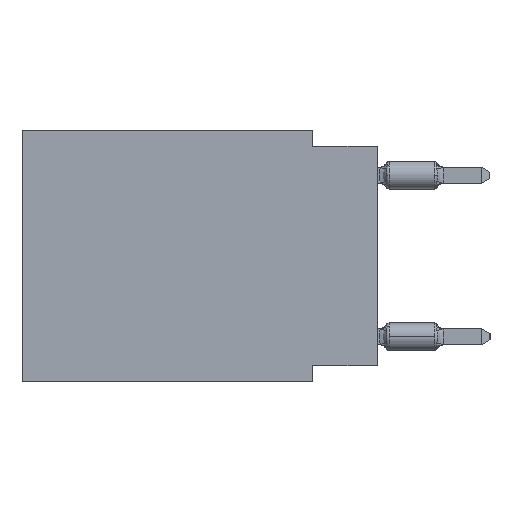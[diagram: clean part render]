
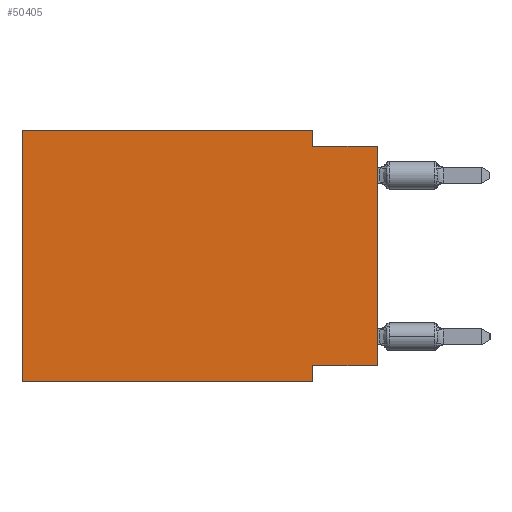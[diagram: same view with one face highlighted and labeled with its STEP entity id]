
A CAD part, left-side view. The second image highlights one B-rep face of the part: STEP entity #50405.
In plain terms, the highlighted planar face has unit normal (-1, 0, 0).
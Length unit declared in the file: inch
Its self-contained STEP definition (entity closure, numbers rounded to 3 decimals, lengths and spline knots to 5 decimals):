
#740 = LINE ( 'NONE', #37298, #24506 ) ;
#2675 = VERTEX_POINT ( 'NONE', #20444 ) ;
#2811 = LINE ( 'NONE', #47509, #9382 ) ;
#3661 = VECTOR ( 'NONE', #38894, 39.37008 ) ;
#3793 = AXIS2_PLACEMENT_3D ( 'NONE', #50603, #45215, #8955 ) ;
#4601 = CARTESIAN_POINT ( 'NONE',  ( 0., 0.1, -0.365 ) ) ;
#4885 = ORIENTED_EDGE ( 'NONE', *, *, #9253, .F. ) ;
#5170 = VERTEX_POINT ( 'NONE', #11547 ) ;
#7883 = CARTESIAN_POINT ( 'NONE',  ( 0., 0.55, -0.39 ) ) ;
#8901 = CARTESIAN_POINT ( 'NONE',  ( 0., 0.1, -0.39 ) ) ;
#8955 = DIRECTION ( 'NONE',  ( 0., 0., -1. ) ) ;
#9253 = EDGE_CURVE ( 'NONE', #12765, #47772, #740, .T. ) ;
#9382 = VECTOR ( 'NONE', #33998, 39.37008 ) ;
#9494 = CARTESIAN_POINT ( 'NONE',  ( 0., 0.1, -0.025 ) ) ;
#11457 = EDGE_CURVE ( 'NONE', #49634, #58229, #49666, .T. ) ;
#11547 = CARTESIAN_POINT ( 'NONE',  ( 0., 0.1, 0. ) ) ;
#11613 = LINE ( 'NONE', #34095, #3661 ) ;
#12765 = VERTEX_POINT ( 'NONE', #9494 ) ;
#13258 = ORIENTED_EDGE ( 'NONE', *, *, #39959, .F. ) ;
#14235 = DIRECTION ( 'NONE',  ( 0., -1., 0. ) ) ;
#15120 = ORIENTED_EDGE ( 'NONE', *, *, #53419, .F. ) ;
#18534 = EDGE_CURVE ( 'NONE', #46167, #5170, #40660, .T. ) ;
#20444 = CARTESIAN_POINT ( 'NONE',  ( 0., 0.55, -0.39 ) ) ;
#20873 = CARTESIAN_POINT ( 'NONE',  ( 0., 0.55, 0. ) ) ;
#21294 = ORIENTED_EDGE ( 'NONE', *, *, #44246, .T. ) ;
#23022 = PLANE ( 'NONE',  #3793 ) ;
#23201 = ORIENTED_EDGE ( 'NONE', *, *, #27641, .F. ) ;
#24506 = VECTOR ( 'NONE', #14235, 39.37008 ) ;
#27139 = DIRECTION ( 'NONE',  ( 0., 0., 1. ) ) ;
#27172 = DIRECTION ( 'NONE',  ( 0., 0., -1. ) ) ;
#27641 = EDGE_CURVE ( 'NONE', #5170, #12765, #2811, .T. ) ;
#27759 = DIRECTION ( 'NONE',  ( 0., -1., 0. ) ) ;
#29787 = VERTEX_POINT ( 'NONE', #34745 ) ;
#32977 = CARTESIAN_POINT ( 'NONE',  ( 0., 0.1, -0.39 ) ) ;
#33998 = DIRECTION ( 'NONE',  ( 0., 0., -1. ) ) ;
#34095 = CARTESIAN_POINT ( 'NONE',  ( 0., 0., 0. ) ) ;
#34745 = CARTESIAN_POINT ( 'NONE',  ( 0., 0., -0.365 ) ) ;
#35008 = VECTOR ( 'NONE', #27759, 39.37008 ) ;
#35621 = EDGE_LOOP ( 'NONE', ( #46133, #4885, #23201, #52230, #15120, #21294, #41038, #13258 ) ) ;
#36783 = LINE ( 'NONE', #54184, #41417 ) ;
#37165 = VECTOR ( 'NONE', #27139, 39.37008 ) ;
#37298 = CARTESIAN_POINT ( 'NONE',  ( 0., 0., -0.025 ) ) ;
#38894 = DIRECTION ( 'NONE',  ( 0., 0., 1. ) ) ;
#39959 = EDGE_CURVE ( 'NONE', #29787, #49634, #36783, .T. ) ;
#40641 = LINE ( 'NONE', #44236, #37165 ) ;
#40660 = LINE ( 'NONE', #49955, #35008 ) ;
#41038 = ORIENTED_EDGE ( 'NONE', *, *, #11457, .F. ) ;
#41417 = VECTOR ( 'NONE', #58960, 39.37008 ) ;
#44236 = CARTESIAN_POINT ( 'NONE',  ( 0., 0.55, 0. ) ) ;
#44246 = EDGE_CURVE ( 'NONE', #2675, #58229, #48945, .T. ) ;
#44920 = FACE_OUTER_BOUND ( 'NONE', #35621, .T. ) ;
#45215 = DIRECTION ( 'NONE',  ( 1., 0., 0. ) ) ;
#46133 = ORIENTED_EDGE ( 'NONE', *, *, #49031, .T. ) ;
#46167 = VERTEX_POINT ( 'NONE', #20873 ) ;
#47509 = CARTESIAN_POINT ( 'NONE',  ( 0., 0.1, 0. ) ) ;
#47772 = VERTEX_POINT ( 'NONE', #58259 ) ;
#48945 = LINE ( 'NONE', #7883, #55147 ) ;
#49031 = EDGE_CURVE ( 'NONE', #29787, #47772, #11613, .T. ) ;
#49634 = VERTEX_POINT ( 'NONE', #4601 ) ;
#49666 = LINE ( 'NONE', #8901, #50854 ) ;
#49955 = CARTESIAN_POINT ( 'NONE',  ( 0., 0.55, 0. ) ) ;
#50405 = ADVANCED_FACE ( 'NONE', ( #44920 ), #23022, .F. ) ;
#50603 = CARTESIAN_POINT ( 'NONE',  ( 0., 0.55, 0. ) ) ;
#50854 = VECTOR ( 'NONE', #27172, 39.37008 ) ;
#52230 = ORIENTED_EDGE ( 'NONE', *, *, #18534, .F. ) ;
#53140 = DIRECTION ( 'NONE',  ( 0., -1., 0. ) ) ;
#53419 = EDGE_CURVE ( 'NONE', #2675, #46167, #40641, .T. ) ;
#54184 = CARTESIAN_POINT ( 'NONE',  ( 0., 0., -0.365 ) ) ;
#55147 = VECTOR ( 'NONE', #53140, 39.37008 ) ;
#58229 = VERTEX_POINT ( 'NONE', #32977 ) ;
#58259 = CARTESIAN_POINT ( 'NONE',  ( 0., 0., -0.025 ) ) ;
#58960 = DIRECTION ( 'NONE',  ( 0., 1., 0. ) ) ;
